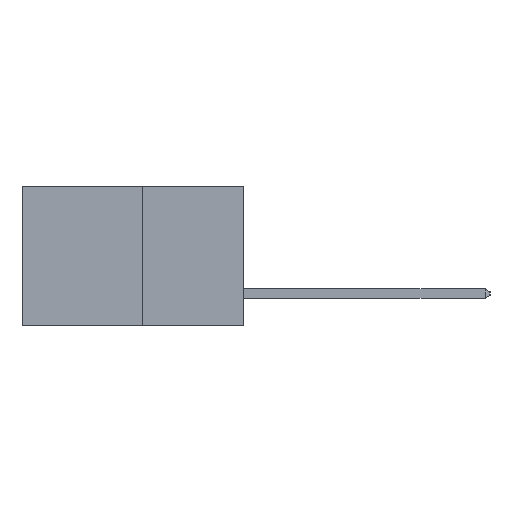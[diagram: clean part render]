
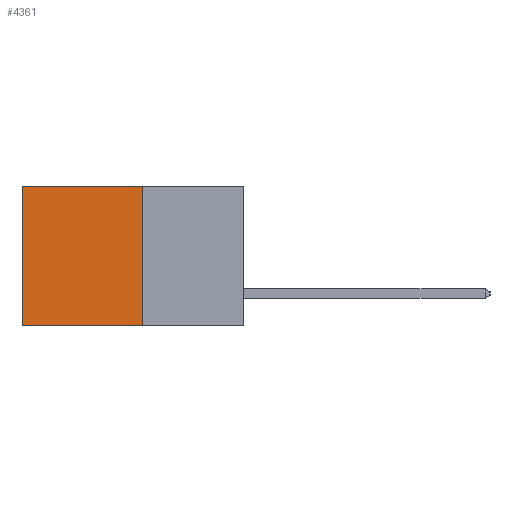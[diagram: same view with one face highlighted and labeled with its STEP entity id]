
A CAD part, left-side view. The second image highlights one B-rep face of the part: STEP entity #4361.
In plain terms, the highlighted planar face has unit normal (-1, 0, 0).
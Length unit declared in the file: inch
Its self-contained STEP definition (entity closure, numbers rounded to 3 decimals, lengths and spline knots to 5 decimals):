
#1 = ORIENTED_EDGE ( 'NONE', *, *, #17166, .F. ) ;
#22 = EDGE_CURVE ( 'NONE', #7393, #18713, #3014, .T. ) ;
#263 = EDGE_LOOP ( 'NONE', ( #11596, #1, #497, #553 ) ) ;
#497 = ORIENTED_EDGE ( 'NONE', *, *, #4787, .F. ) ;
#553 = ORIENTED_EDGE ( 'NONE', *, *, #6621, .T. ) ;
#666 = DIRECTION ( 'NONE',  ( 0., 0., -1. ) ) ;
#2984 = CARTESIAN_POINT ( 'NONE',  ( 0.277, 0.27, 0. ) ) ;
#3014 = LINE ( 'NONE', #14005, #18441 ) ;
#4361 = ADVANCED_FACE ( 'NONE', ( #17889 ), #14861, .F. ) ;
#4509 = DIRECTION ( 'NONE',  ( 0., 1., 0. ) ) ;
#4787 = EDGE_CURVE ( 'NONE', #12876, #6605, #6537, .T. ) ;
#6537 = LINE ( 'NONE', #8506, #18354 ) ;
#6605 = VERTEX_POINT ( 'NONE', #18333 ) ;
#6621 = EDGE_CURVE ( 'NONE', #12876, #7393, #18965, .T. ) ;
#7065 = CARTESIAN_POINT ( 'NONE',  ( 0.277, 0.27, -0.37 ) ) ;
#7393 = VERTEX_POINT ( 'NONE', #8144 ) ;
#8144 = CARTESIAN_POINT ( 'NONE',  ( 0.277, 0.59, 0. ) ) ;
#8506 = CARTESIAN_POINT ( 'NONE',  ( 0.277, 0.27, -0.37 ) ) ;
#8659 = DIRECTION ( 'NONE',  ( 0., 0., -1. ) ) ;
#9966 = CARTESIAN_POINT ( 'NONE',  ( 0.277, 0.27, 0. ) ) ;
#10928 = VECTOR ( 'NONE', #4509, 39.37008 ) ;
#11596 = ORIENTED_EDGE ( 'NONE', *, *, #22, .T. ) ;
#11672 = DIRECTION ( 'NONE',  ( 0., 1., 0. ) ) ;
#12699 = LINE ( 'NONE', #19190, #15780 ) ;
#12876 = VERTEX_POINT ( 'NONE', #9966 ) ;
#14005 = CARTESIAN_POINT ( 'NONE',  ( 0.277, 0.59, -0.37 ) ) ;
#14044 = AXIS2_PLACEMENT_3D ( 'NONE', #7065, #17862, #8659 ) ;
#14116 = DIRECTION ( 'NONE',  ( 0., 0., -1. ) ) ;
#14861 = PLANE ( 'NONE',  #14044 ) ;
#15780 = VECTOR ( 'NONE', #11672, 39.37008 ) ;
#17166 = EDGE_CURVE ( 'NONE', #6605, #18713, #12699, .T. ) ;
#17862 = DIRECTION ( 'NONE',  ( 1., 0., 0. ) ) ;
#17889 = FACE_OUTER_BOUND ( 'NONE', #263, .T. ) ;
#18305 = CARTESIAN_POINT ( 'NONE',  ( 0.277, 0.59, -0.37 ) ) ;
#18333 = CARTESIAN_POINT ( 'NONE',  ( 0.277, 0.27, -0.37 ) ) ;
#18354 = VECTOR ( 'NONE', #666, 39.37008 ) ;
#18441 = VECTOR ( 'NONE', #14116, 39.37008 ) ;
#18713 = VERTEX_POINT ( 'NONE', #18305 ) ;
#18965 = LINE ( 'NONE', #2984, #10928 ) ;
#19190 = CARTESIAN_POINT ( 'NONE',  ( 0.277, 0.27, -0.37 ) ) ;
